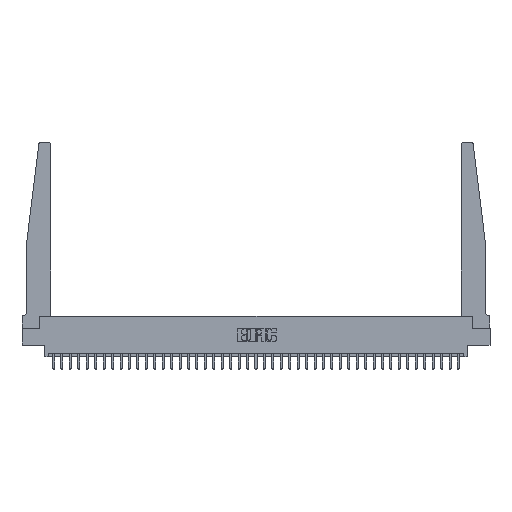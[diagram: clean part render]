
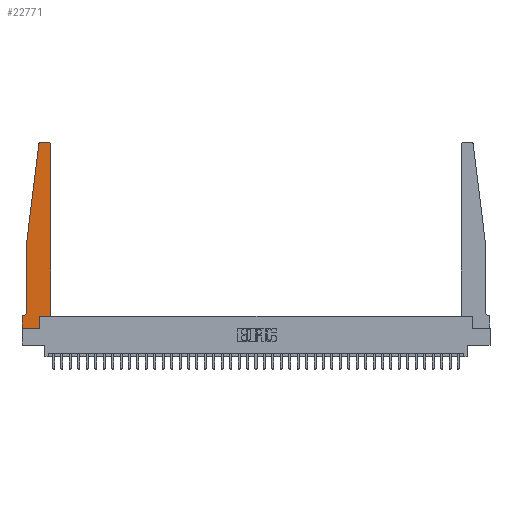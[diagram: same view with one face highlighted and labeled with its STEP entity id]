
A CAD part, top view. The second image highlights one B-rep face of the part: STEP entity #22771.
In plain terms, the highlighted planar face has unit normal (0, 0, 1).
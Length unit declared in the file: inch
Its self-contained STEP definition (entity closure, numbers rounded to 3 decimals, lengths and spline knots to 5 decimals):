
#34 = VERTEX_POINT ( 'NONE', #5906 ) ;
#305 = ORIENTED_EDGE ( 'NONE', *, *, #35378, .T. ) ;
#312 = VERTEX_POINT ( 'NONE', #22375 ) ;
#1270 = EDGE_CURVE ( 'NONE', #35515, #4832, #15321, .T. ) ;
#1288 = VECTOR ( 'NONE', #34814, 39.37008 ) ;
#1844 = CARTESIAN_POINT ( 'NONE',  ( 0.425, 0.18, 0.37 ) ) ;
#2063 = AXIS2_PLACEMENT_3D ( 'NONE', #4606, #24169, #7434 ) ;
#2074 = DIRECTION ( 'NONE',  ( 0., 0., 1. ) ) ;
#2096 = DIRECTION ( 'NONE',  ( 0., 0., 1. ) ) ;
#2728 = ORIENTED_EDGE ( 'NONE', *, *, #33553, .T. ) ;
#2741 = DIRECTION ( 'NONE',  ( -1., 0., 0. ) ) ;
#3442 = DIRECTION ( 'NONE',  ( -1., 0., 0. ) ) ;
#4198 = VECTOR ( 'NONE', #10983, 39.37008 ) ;
#4450 = ORIENTED_EDGE ( 'NONE', *, *, #19058, .T. ) ;
#4498 = CARTESIAN_POINT ( 'NONE',  ( 0., 0.1875, 0.37 ) ) ;
#4606 = CARTESIAN_POINT ( 'NONE',  ( 0.015, 0.2375, 0.37 ) ) ;
#4832 = VERTEX_POINT ( 'NONE', #19852 ) ;
#4953 = AXIS2_PLACEMENT_3D ( 'NONE', #18892, #2074, #21715 ) ;
#5906 = CARTESIAN_POINT ( 'NONE',  ( 0.425, 0.18, 0.37 ) ) ;
#5939 = AXIS2_PLACEMENT_3D ( 'NONE', #29758, #13099, #32498 ) ;
#6795 = CARTESIAN_POINT ( 'NONE',  ( 0.2605, 0.18, 0.37 ) ) ;
#6979 = CARTESIAN_POINT ( 'NONE',  ( 0., 0., 0.37 ) ) ;
#7376 = ORIENTED_EDGE ( 'NONE', *, *, #35368, .T. ) ;
#7434 = DIRECTION ( 'NONE',  ( -1., 0., 0. ) ) ;
#7473 = ORIENTED_EDGE ( 'NONE', *, *, #18335, .T. ) ;
#7515 = LINE ( 'NONE', #1844, #8378 ) ;
#8378 = VECTOR ( 'NONE', #15995, 39.37008 ) ;
#8778 = LINE ( 'NONE', #9361, #16204 ) ;
#9361 = CARTESIAN_POINT ( 'NONE',  ( 0., 0., 0.37 ) ) ;
#10114 = CARTESIAN_POINT ( 'NONE',  ( 0.2605, 0.18, 0.37 ) ) ;
#10246 = DIRECTION ( 'NONE',  ( 0., 1., 0. ) ) ;
#10323 = LINE ( 'NONE', #16719, #24321 ) ;
#10499 = PLANE ( 'NONE',  #4953 ) ;
#10513 = ORIENTED_EDGE ( 'NONE', *, *, #14506, .T. ) ;
#10983 = DIRECTION ( 'NONE',  ( 0., -1., 0. ) ) ;
#11529 = VERTEX_POINT ( 'NONE', #6979 ) ;
#11816 = EDGE_CURVE ( 'NONE', #11932, #31998, #32935, .T. ) ;
#11932 = VERTEX_POINT ( 'NONE', #20104 ) ;
#12229 = VERTEX_POINT ( 'NONE', #15836 ) ;
#13099 = DIRECTION ( 'NONE',  ( 0., 0., 1. ) ) ;
#13519 = CARTESIAN_POINT ( 'NONE',  ( 0.24675, 2.72367, 0.37 ) ) ;
#14506 = EDGE_CURVE ( 'NONE', #12229, #32502, #16806, .T. ) ;
#14635 = DIRECTION ( 'NONE',  ( 1., 0., 0. ) ) ;
#14969 = LINE ( 'NONE', #10114, #16258 ) ;
#15321 = CIRCLE ( 'NONE', #19395, 0.03 ) ;
#15836 = CARTESIAN_POINT ( 'NONE',  ( 0.27653, 2.75, 0.37 ) ) ;
#15995 = DIRECTION ( 'NONE',  ( 0., 1., 0. ) ) ;
#16204 = VECTOR ( 'NONE', #23314, 39.37008 ) ;
#16258 = VECTOR ( 'NONE', #10246, 39.37008 ) ;
#16416 = ORIENTED_EDGE ( 'NONE', *, *, #32423, .T. ) ;
#16719 = CARTESIAN_POINT ( 'NONE',  ( 0.065, 0.1875, 0.37 ) ) ;
#16806 = CIRCLE ( 'NONE', #5939, 0.03 ) ;
#17175 = CARTESIAN_POINT ( 'NONE',  ( 0.065, 1.25, 0.37 ) ) ;
#17521 = EDGE_CURVE ( 'NONE', #34, #35515, #7515, .T. ) ;
#17643 = CARTESIAN_POINT ( 'NONE',  ( 0., 0., 0.37 ) ) ;
#18324 = LINE ( 'NONE', #17175, #25807 ) ;
#18335 = EDGE_CURVE ( 'NONE', #32502, #11932, #18324, .T. ) ;
#18413 = CARTESIAN_POINT ( 'NONE',  ( 0.2605, 0., 0.37 ) ) ;
#18892 = CARTESIAN_POINT ( 'NONE',  ( 0., 0.1875, 0.37 ) ) ;
#18913 = CARTESIAN_POINT ( 'NONE',  ( 0.395, 2.72, 0.37 ) ) ;
#19058 = EDGE_CURVE ( 'NONE', #4832, #12229, #27897, .T. ) ;
#19395 = AXIS2_PLACEMENT_3D ( 'NONE', #18913, #2096, #21735 ) ;
#19852 = CARTESIAN_POINT ( 'NONE',  ( 0.395, 2.75, 0.37 ) ) ;
#20101 = EDGE_CURVE ( 'NONE', #312, #22635, #10323, .T. ) ;
#20104 = CARTESIAN_POINT ( 'NONE',  ( 0.065, 1.25, 0.37 ) ) ;
#20468 = VECTOR ( 'NONE', #3442, 39.37008 ) ;
#21715 = DIRECTION ( 'NONE',  ( 1., 0., 0. ) ) ;
#21735 = DIRECTION ( 'NONE',  ( 1., 0., 0. ) ) ;
#22375 = CARTESIAN_POINT ( 'NONE',  ( 0.015, 0.1875, 0.37 ) ) ;
#22635 = VERTEX_POINT ( 'NONE', #4498 ) ;
#22771 = ADVANCED_FACE ( 'NONE', ( #25061 ), #10499, .T. ) ;
#23102 = ORIENTED_EDGE ( 'NONE', *, *, #1270, .T. ) ;
#23314 = DIRECTION ( 'NONE',  ( 0., -1., 0. ) ) ;
#23721 = LINE ( 'NONE', #26594, #1288 ) ;
#23767 = ORIENTED_EDGE ( 'NONE', *, *, #17521, .T. ) ;
#23942 = ORIENTED_EDGE ( 'NONE', *, *, #20101, .T. ) ;
#24169 = DIRECTION ( 'NONE',  ( 0., 0., -1. ) ) ;
#24321 = VECTOR ( 'NONE', #2741, 39.37008 ) ;
#24552 = VECTOR ( 'NONE', #14635, 39.37008 ) ;
#24970 = CIRCLE ( 'NONE', #2063, 0.05 ) ;
#25044 = ORIENTED_EDGE ( 'NONE', *, *, #35586, .T. ) ;
#25061 = FACE_OUTER_BOUND ( 'NONE', #25943, .T. ) ;
#25807 = VECTOR ( 'NONE', #31056, 39.37008 ) ;
#25943 = EDGE_LOOP ( 'NONE', ( #4450, #10513, #7473, #30192, #25044, #23942, #305, #7376, #2728, #16416, #23767, #23102 ) ) ;
#26594 = CARTESIAN_POINT ( 'NONE',  ( 0.425, 0.18, 0.37 ) ) ;
#26618 = CARTESIAN_POINT ( 'NONE',  ( 0.425, 2.72, 0.37 ) ) ;
#27660 = VERTEX_POINT ( 'NONE', #6795 ) ;
#27686 = CARTESIAN_POINT ( 'NONE',  ( 0.065, 1.25, 0.37 ) ) ;
#27897 = LINE ( 'NONE', #31251, #20468 ) ;
#29758 = CARTESIAN_POINT ( 'NONE',  ( 0.27653, 2.72, 0.37 ) ) ;
#30192 = ORIENTED_EDGE ( 'NONE', *, *, #11816, .T. ) ;
#30206 = CARTESIAN_POINT ( 'NONE',  ( 0.065, 0.2375, 0.37 ) ) ;
#31056 = DIRECTION ( 'NONE',  ( -0.122, -0.992, 0. ) ) ;
#31251 = CARTESIAN_POINT ( 'NONE',  ( 0.25, 2.75, 0.37 ) ) ;
#31855 = LINE ( 'NONE', #17643, #24552 ) ;
#31998 = VERTEX_POINT ( 'NONE', #30206 ) ;
#32423 = EDGE_CURVE ( 'NONE', #27660, #34, #23721, .T. ) ;
#32498 = DIRECTION ( 'NONE',  ( 1., 0., 0. ) ) ;
#32502 = VERTEX_POINT ( 'NONE', #13519 ) ;
#32935 = LINE ( 'NONE', #27686, #4198 ) ;
#33553 = EDGE_CURVE ( 'NONE', #34890, #27660, #14969, .T. ) ;
#34814 = DIRECTION ( 'NONE',  ( 1., 0., 0. ) ) ;
#34890 = VERTEX_POINT ( 'NONE', #18413 ) ;
#35368 = EDGE_CURVE ( 'NONE', #11529, #34890, #31855, .T. ) ;
#35378 = EDGE_CURVE ( 'NONE', #22635, #11529, #8778, .T. ) ;
#35515 = VERTEX_POINT ( 'NONE', #26618 ) ;
#35586 = EDGE_CURVE ( 'NONE', #31998, #312, #24970, .T. ) ;
